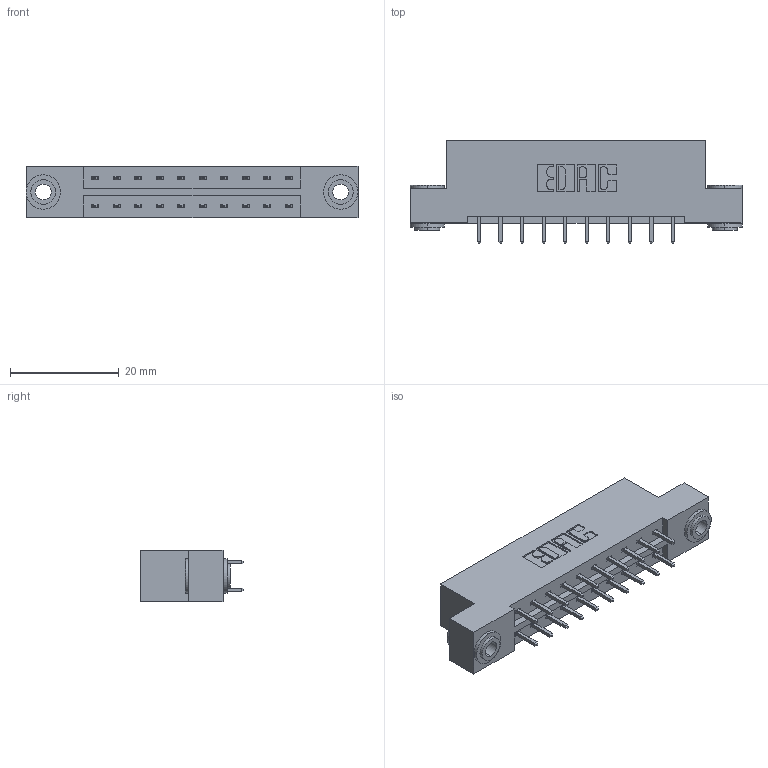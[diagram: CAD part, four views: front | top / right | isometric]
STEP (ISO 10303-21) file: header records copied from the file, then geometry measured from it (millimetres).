
FILE_DESCRIPTION (( 'STEP AP203' ), '1' );
FILE_NAME ('333-020-521-203.STEP', '2018-08-01T23:43:01', ( '' ), ( '' ), 'SwSTEP 2.0', 'SolidWorks 2016', '' );
FILE_SCHEMA (( 'CONFIG_CONTROL_DESIGN' ));
Length unit declared in the file: inch
Products named in the file (4): 333-020-521-203; 333 Part_Flush - .156 Dia - TH; 345-292-001_345-293-121; 345-250-002_345-250-002-102
Assembly tree (23 placements, depth 2):
  333-020-521-203
    333 Part_Flush - .156 Dia - TH
    345-292-001_345-293-121  x20
    345-250-002_345-250-002-102  x2
Bounding box: 61.16 x 19.06 x 9.4 mm (x, y, z)
Volume: 5956.4 mm3; surface area: 6861.4 mm2
Topology: 23 solids, 23 shells, 1192 faces, 3487 edges, 2294 vertices
Faces by surface type: plane 800, cylinder 384, cone 8
Entity records: 11240 total; most frequent: CARTESIAN_POINT 1877, ORIENTED_EDGE 1806, DIRECTION 1693, EDGE_CURVE 903, VECTOR 751, LINE 751, VERTEX_POINT 598, AXIS2_PLACEMENT_3D 471
